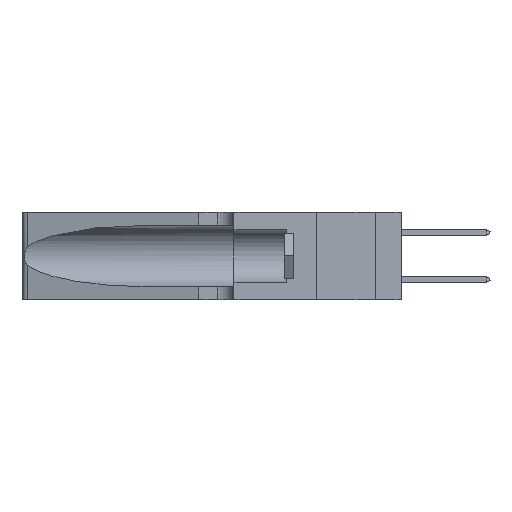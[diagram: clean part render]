
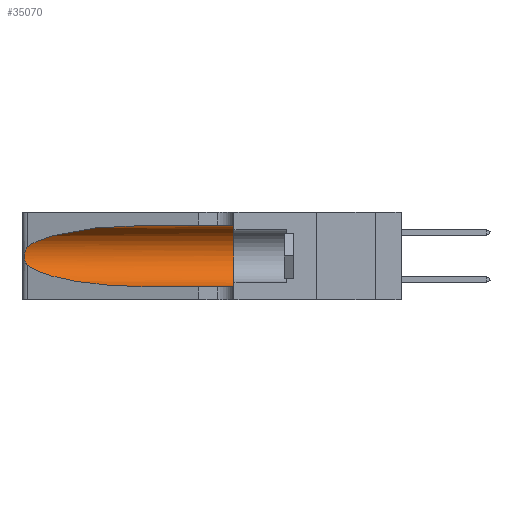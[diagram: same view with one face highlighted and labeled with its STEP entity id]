
A CAD part, left-side view. The second image highlights one B-rep face of the part: STEP entity #35070.
In plain terms, the highlighted cylindrical face has radius 3.308 mm (diameter 6.617 mm), a partial arc.
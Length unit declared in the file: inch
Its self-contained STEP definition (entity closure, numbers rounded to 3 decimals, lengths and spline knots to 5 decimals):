
#758 = VERTEX_POINT ( 'NONE', #10340 ) ;
#2680 = LINE ( 'NONE', #20709, #19353 ) ;
#2786 = CARTESIAN_POINT ( 'NONE',  ( 0.1305, 0.35, 0.05475 ) ) ;
#3181 = CARTESIAN_POINT ( 'NONE',  ( 0.26075, 1.23896, 0.178 ) ) ;
#3625 =( BOUNDED_CURVE ( )  B_SPLINE_CURVE ( 3, ( #21403, #41282, #4802, #28071 ),
 .UNSPECIFIED., .F., .T. ) 
 B_SPLINE_CURVE_WITH_KNOTS ( ( 4, 4 ),
 ( 3.44316, 4.71239 ),
 .UNSPECIFIED. ) 
 CURVE ( )  GEOMETRIC_REPRESENTATION_ITEM ( )  RATIONAL_B_SPLINE_CURVE ( ( 1., 0.87, 0.87, 1. ) ) 
 REPRESENTATION_ITEM ( '' )  );
#4161 = VECTOR ( 'NONE', #34861, 39.37008 ) ;
#4802 = CARTESIAN_POINT ( 'NONE',  ( 0.18966, 0.96281, 0.05475 ) ) ;
#5120 = DIRECTION ( 'NONE',  ( 0., 0., -1. ) ) ;
#5325 = ORIENTED_EDGE ( 'NONE', *, *, #21327, .F. ) ;
#6245 = CARTESIAN_POINT ( 'NONE',  ( 0.25487, 1.22718, 0.22369 ) ) ;
#6395 = CARTESIAN_POINT ( 'NONE',  ( 0.25555, 1.22994, 0.2215 ) ) ;
#6542 = CARTESIAN_POINT ( 'NONE',  ( 0.25856, 1.23593, 0.16098 ) ) ;
#8503 = CARTESIAN_POINT ( 'NONE',  ( 0.1305, 1.61858, 0.185 ) ) ;
#9535 = VERTEX_POINT ( 'NONE', #12348 ) ;
#9610 = EDGE_CURVE ( 'NONE', #41042, #758, #26838, .T. ) ;
#9622 = EDGE_CURVE ( 'NONE', #758, #9535, #19116, .T. ) ;
#9883 = CARTESIAN_POINT ( 'NONE',  ( 0.25639, 1.23186, 0.15144 ) ) ;
#10340 = CARTESIAN_POINT ( 'NONE',  ( 0.25487, 1.22718, 0.22369 ) ) ;
#11000 = CYLINDRICAL_SURFACE ( 'NONE', #19191, 0.13025 ) ;
#12100 = ORIENTED_EDGE ( 'NONE', *, *, #9622, .T. ) ;
#12348 = CARTESIAN_POINT ( 'NONE',  ( 0.25487, 1.22718, 0.14631 ) ) ;
#12994 = LINE ( 'NONE', #31518, #4161 ) ;
#13140 = ORIENTED_EDGE ( 'NONE', *, *, #34832, .T. ) ;
#13230 = CARTESIAN_POINT ( 'NONE',  ( 0.25487, 1.22718, 0.14631 ) ) ;
#15613 = EDGE_CURVE ( 'NONE', #9535, #25453, #3625, .T. ) ;
#16440 = CARTESIAN_POINT ( 'NONE',  ( 0.25639, 1.23184, 0.21858 ) ) ;
#18836 = DIRECTION ( 'NONE',  ( 0., 1., 0. ) ) ;
#19116 = B_SPLINE_CURVE_WITH_KNOTS ( 'NONE', 3,
 ( #29641, #6395, #16440, #39668, #19768, #43022, #23134, #3181, #26462, #6542, #29785, #9883, #33153, #13230 ),
 .UNSPECIFIED., .F., .F.,
 ( 4, 2, 2, 2, 2, 2, 4 ),
 ( 0., 0.00027, 0.00053, 0.00107, 0.0016, 0.00187, 0.00214 ),
 .UNSPECIFIED. ) ;
#19191 = AXIS2_PLACEMENT_3D ( 'NONE', #8503, #35080, #5120 ) ;
#19353 = VECTOR ( 'NONE', #24065, 39.37008 ) ;
#19768 = CARTESIAN_POINT ( 'NONE',  ( 0.25854, 1.2359, 0.20912 ) ) ;
#20709 = CARTESIAN_POINT ( 'NONE',  ( 0.1305, 1.61858, 0.05475 ) ) ;
#20904 = FACE_OUTER_BOUND ( 'NONE', #36941, .T. ) ;
#21327 = EDGE_CURVE ( 'NONE', #21725, #27662, #29812, .T. ) ;
#21403 = CARTESIAN_POINT ( 'NONE',  ( 0.25487, 1.22718, 0.14631 ) ) ;
#21725 = VERTEX_POINT ( 'NONE', #24486 ) ;
#23134 = CARTESIAN_POINT ( 'NONE',  ( 0.26075, 1.23896, 0.19203 ) ) ;
#23527 = ORIENTED_EDGE ( 'NONE', *, *, #28752, .F. ) ;
#24065 = DIRECTION ( 'NONE',  ( 0., -1., 0. ) ) ;
#24486 = CARTESIAN_POINT ( 'NONE',  ( 0.1305, 0.35, 0.31525 ) ) ;
#25453 = VERTEX_POINT ( 'NONE', #28036 ) ;
#26192 = CARTESIAN_POINT ( 'NONE',  ( 0.2373, 1.15595, 0.28018 ) ) ;
#26462 = CARTESIAN_POINT ( 'NONE',  ( 0.26017, 1.23833, 0.17102 ) ) ;
#26838 =( BOUNDED_CURVE ( )  B_SPLINE_CURVE ( 3, ( #42747, #39240, #26192, #6245 ),
 .UNSPECIFIED., .F., .T. ) 
 B_SPLINE_CURVE_WITH_KNOTS ( ( 4, 4 ),
 ( 1.5708, 2.84003 ),
 .UNSPECIFIED. ) 
 CURVE ( )  GEOMETRIC_REPRESENTATION_ITEM ( )  RATIONAL_B_SPLINE_CURVE ( ( 1., 0.87, 0.87, 1. ) ) 
 REPRESENTATION_ITEM ( '' )  );
#27662 = VERTEX_POINT ( 'NONE', #2786 ) ;
#27725 = CARTESIAN_POINT ( 'NONE',  ( 0.1305, 0.72297, 0.31525 ) ) ;
#28036 = CARTESIAN_POINT ( 'NONE',  ( 0.1305, 0.72297, 0.05475 ) ) ;
#28071 = CARTESIAN_POINT ( 'NONE',  ( 0.1305, 0.72297, 0.05475 ) ) ;
#28752 = EDGE_CURVE ( 'NONE', #41042, #21725, #12994, .T. ) ;
#29641 = CARTESIAN_POINT ( 'NONE',  ( 0.25487, 1.22718, 0.22369 ) ) ;
#29785 = CARTESIAN_POINT ( 'NONE',  ( 0.25789, 1.23486, 0.15765 ) ) ;
#29812 = CIRCLE ( 'NONE', #42796, 0.13025 ) ;
#29960 = ORIENTED_EDGE ( 'NONE', *, *, #15613, .T. ) ;
#31518 = CARTESIAN_POINT ( 'NONE',  ( 0.1305, 1.61858, 0.31525 ) ) ;
#33153 = CARTESIAN_POINT ( 'NONE',  ( 0.25555, 1.22993, 0.14849 ) ) ;
#34832 = EDGE_CURVE ( 'NONE', #25453, #27662, #2680, .T. ) ;
#34861 = DIRECTION ( 'NONE',  ( 0., -1., 0. ) ) ;
#35070 = ADVANCED_FACE ( 'NONE', ( #20904 ), #11000, .F. ) ;
#35080 = DIRECTION ( 'NONE',  ( 0., -1., 0. ) ) ;
#36941 = EDGE_LOOP ( 'NONE', ( #38309, #12100, #29960, #13140, #5325, #23527 ) ) ;
#38309 = ORIENTED_EDGE ( 'NONE', *, *, #9610, .T. ) ;
#38718 = CARTESIAN_POINT ( 'NONE',  ( 0.1305, 0.35, 0.185 ) ) ;
#39240 = CARTESIAN_POINT ( 'NONE',  ( 0.18966, 0.96281, 0.31525 ) ) ;
#39668 = CARTESIAN_POINT ( 'NONE',  ( 0.25787, 1.23484, 0.2124 ) ) ;
#41042 = VERTEX_POINT ( 'NONE', #27725 ) ;
#41282 = CARTESIAN_POINT ( 'NONE',  ( 0.2373, 1.15595, 0.08982 ) ) ;
#42054 = DIRECTION ( 'NONE',  ( 0., 0., 1. ) ) ;
#42747 = CARTESIAN_POINT ( 'NONE',  ( 0.1305, 0.72297, 0.31525 ) ) ;
#42796 = AXIS2_PLACEMENT_3D ( 'NONE', #38718, #18836, #42054 ) ;
#43022 = CARTESIAN_POINT ( 'NONE',  ( 0.26018, 1.23835, 0.19895 ) ) ;
